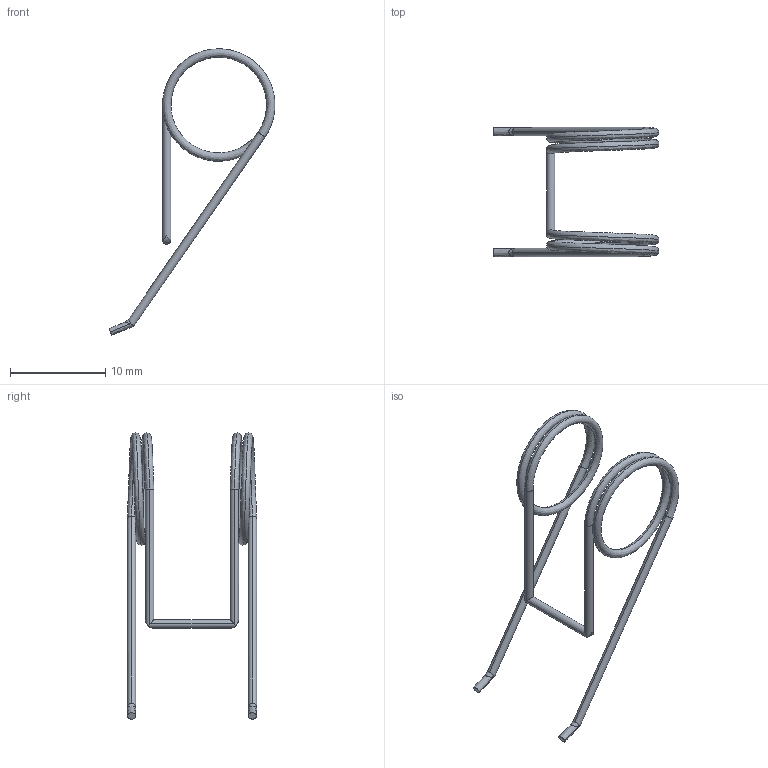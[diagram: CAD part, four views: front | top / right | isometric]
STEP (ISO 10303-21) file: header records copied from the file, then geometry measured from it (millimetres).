
FILE_DESCRIPTION (( 'STEP AP214' ), '1' );
FILE_NAME ('Trigger Spring.step.step', '2019-12-18T03:08:55', ( '' ), ( '' ), 'SwSTEP 2.0', 'SolidWorks 2019', '' );
FILE_SCHEMA (( 'AUTOMOTIVE_DESIGN' ));
Length unit declared in the file: millimetre
Products named in the file (1): Trigger Spring.step
Bounding box: 17.42 x 13.59 x 30.07 mm (x, y, z)
Volume: 123.3 mm3; surface area: 557 mm2
Topology: 1 solids, 1 shells, 24 faces, 61 edges, 37 vertices
Faces by surface type: cylinder 12, bspline 10, plane 2
Entity records: 2090 total; most frequent: CARTESIAN_POINT 1620, ORIENTED_EDGE 118, EDGE_CURVE 59, DIRECTION 48, VERTEX_POINT 37, B_SPLINE_CURVE_WITH_KNOTS 35, FACE_OUTER_BOUND 24, EDGE_LOOP 24
